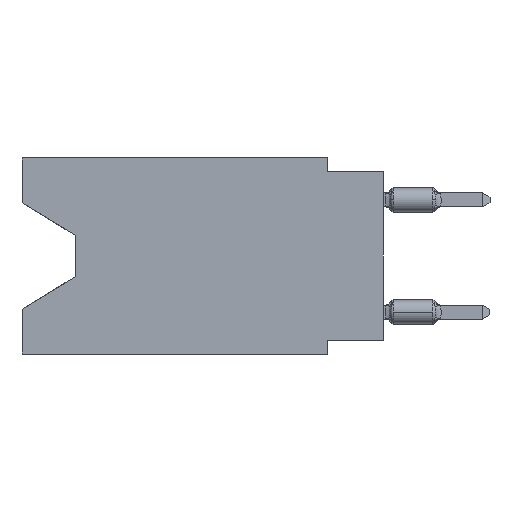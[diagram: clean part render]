
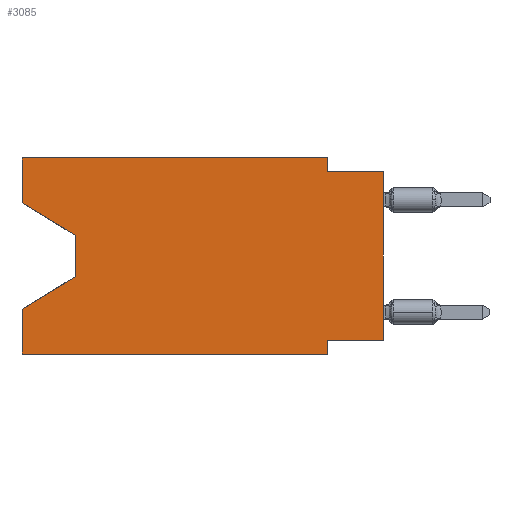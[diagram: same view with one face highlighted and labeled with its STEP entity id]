
A CAD part, left-side view. The second image highlights one B-rep face of the part: STEP entity #3085.
In plain terms, the highlighted planar face has unit normal (-1, 0, 0).
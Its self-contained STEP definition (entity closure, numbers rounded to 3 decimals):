
#282 = ORIENTED_EDGE ( 'NONE', *, *, #13436, .F. ) ;
#720 = LINE ( 'NONE', #1705, #8904 ) ;
#852 = EDGE_CURVE ( 'NONE', #2510, #11657, #2677, .T. ) ;
#994 = CARTESIAN_POINT ( 'NONE',  ( 0., 0., -8.255 ) ) ;
#1095 = LINE ( 'NONE', #13838, #10839 ) ;
#1414 = CARTESIAN_POINT ( 'NONE',  ( 0., 0., -0.635 ) ) ;
#1499 = ORIENTED_EDGE ( 'NONE', *, *, #11887, .F. ) ;
#1631 = ORIENTED_EDGE ( 'NONE', *, *, #2037, .T. ) ;
#1705 = CARTESIAN_POINT ( 'NONE',  ( 0., 16.383, -2.038 ) ) ;
#1725 = DIRECTION ( 'NONE',  ( 0., -1., 0. ) ) ;
#1851 = EDGE_CURVE ( 'NONE', #5161, #9197, #10149, .T. ) ;
#1967 = VERTEX_POINT ( 'NONE', #6021 ) ;
#1979 = DIRECTION ( 'NONE',  ( 0., 0., 1. ) ) ;
#2037 = EDGE_CURVE ( 'NONE', #12470, #5170, #7207, .T. ) ;
#2346 = DIRECTION ( 'NONE',  ( 0., 1., 0. ) ) ;
#2455 = ORIENTED_EDGE ( 'NONE', *, *, #5030, .T. ) ;
#2510 = VERTEX_POINT ( 'NONE', #6070 ) ;
#2540 = DIRECTION ( 'NONE',  ( 0., -1., 0. ) ) ;
#2578 = LINE ( 'NONE', #3625, #4548 ) ;
#2656 = DIRECTION ( 'NONE',  ( 0., 0., 1. ) ) ;
#2677 = LINE ( 'NONE', #13384, #4846 ) ;
#2776 = LINE ( 'NONE', #11307, #4141 ) ;
#2982 = EDGE_CURVE ( 'NONE', #5170, #8091, #7319, .T. ) ;
#3081 = CARTESIAN_POINT ( 'NONE',  ( 0., 16.383, -8.89 ) ) ;
#3085 = ADVANCED_FACE ( 'NONE', ( #8920 ), #7593, .F. ) ;
#3102 = EDGE_CURVE ( 'NONE', #3822, #9197, #7659, .T. ) ;
#3211 = AXIS2_PLACEMENT_3D ( 'NONE', #3523, #10937, #4641 ) ;
#3237 = DIRECTION ( 'NONE',  ( 0., 0., -1. ) ) ;
#3421 = ORIENTED_EDGE ( 'NONE', *, *, #4688, .T. ) ;
#3451 = VECTOR ( 'NONE', #2346, 1000. ) ;
#3523 = CARTESIAN_POINT ( 'NONE',  ( 0., 16.383, 0. ) ) ;
#3625 = CARTESIAN_POINT ( 'NONE',  ( 0., 2.54, -8.89 ) ) ;
#3763 = CARTESIAN_POINT ( 'NONE',  ( 0., 2.54, 0. ) ) ;
#3798 = DIRECTION ( 'NONE',  ( 0., -1., 0. ) ) ;
#3822 = VERTEX_POINT ( 'NONE', #11272 ) ;
#3915 = CARTESIAN_POINT ( 'NONE',  ( 0., 13.97, -3.505 ) ) ;
#4141 = VECTOR ( 'NONE', #1725, 1000. ) ;
#4416 = VERTEX_POINT ( 'NONE', #12717 ) ;
#4548 = VECTOR ( 'NONE', #10003, 1000. ) ;
#4641 = DIRECTION ( 'NONE',  ( 0., 0., -1. ) ) ;
#4688 = EDGE_CURVE ( 'NONE', #6809, #1967, #2776, .T. ) ;
#4715 = VERTEX_POINT ( 'NONE', #6003 ) ;
#4846 = VECTOR ( 'NONE', #3798, 1000. ) ;
#4956 = CARTESIAN_POINT ( 'NONE',  ( 0., 13.97, -3.505 ) ) ;
#5006 = VECTOR ( 'NONE', #2540, 1000. ) ;
#5030 = EDGE_CURVE ( 'NONE', #4715, #12470, #720, .T. ) ;
#5161 = VERTEX_POINT ( 'NONE', #994 ) ;
#5170 = VERTEX_POINT ( 'NONE', #5408 ) ;
#5408 = CARTESIAN_POINT ( 'NONE',  ( 0., 13.97, -5.385 ) ) ;
#5431 = CARTESIAN_POINT ( 'NONE',  ( 0., 0., -8.255 ) ) ;
#6003 = CARTESIAN_POINT ( 'NONE',  ( 0., 16.383, -2.038 ) ) ;
#6021 = CARTESIAN_POINT ( 'NONE',  ( 0., 2.54, -8.89 ) ) ;
#6070 = CARTESIAN_POINT ( 'NONE',  ( 0., 16.383, 0. ) ) ;
#6258 = CARTESIAN_POINT ( 'NONE',  ( 0., 13.97, -5.385 ) ) ;
#6510 = EDGE_CURVE ( 'NONE', #4715, #2510, #9610, .T. ) ;
#6740 = ORIENTED_EDGE ( 'NONE', *, *, #3102, .F. ) ;
#6809 = VERTEX_POINT ( 'NONE', #3081 ) ;
#7001 = CARTESIAN_POINT ( 'NONE',  ( 0., 0., 0. ) ) ;
#7096 = EDGE_CURVE ( 'NONE', #6809, #8091, #1095, .T. ) ;
#7201 = VECTOR ( 'NONE', #3237, 1000. ) ;
#7207 = LINE ( 'NONE', #4956, #12679 ) ;
#7319 = LINE ( 'NONE', #6258, #7476 ) ;
#7476 = VECTOR ( 'NONE', #13807, 1000. ) ;
#7593 = PLANE ( 'NONE',  #3211 ) ;
#7659 = LINE ( 'NONE', #1414, #5006 ) ;
#7849 = EDGE_LOOP ( 'NONE', ( #2455, #1631, #9806, #8907, #3421, #10992, #1499, #8838, #6740, #282, #10157, #9164 ) ) ;
#8091 = VERTEX_POINT ( 'NONE', #9621 ) ;
#8342 = VECTOR ( 'NONE', #2656, 1000. ) ;
#8394 = DIRECTION ( 'NONE',  ( 0., 0., 1. ) ) ;
#8727 = LINE ( 'NONE', #5431, #3451 ) ;
#8838 = ORIENTED_EDGE ( 'NONE', *, *, #1851, .T. ) ;
#8904 = VECTOR ( 'NONE', #10383, 1000. ) ;
#8907 = ORIENTED_EDGE ( 'NONE', *, *, #7096, .F. ) ;
#8920 = FACE_OUTER_BOUND ( 'NONE', #7849, .T. ) ;
#9164 = ORIENTED_EDGE ( 'NONE', *, *, #6510, .F. ) ;
#9197 = VERTEX_POINT ( 'NONE', #12702 ) ;
#9610 = LINE ( 'NONE', #11566, #10171 ) ;
#9621 = CARTESIAN_POINT ( 'NONE',  ( 0., 16.383, -6.852 ) ) ;
#9806 = ORIENTED_EDGE ( 'NONE', *, *, #2982, .T. ) ;
#10003 = DIRECTION ( 'NONE',  ( 0., 0., -1. ) ) ;
#10149 = LINE ( 'NONE', #7001, #8342 ) ;
#10157 = ORIENTED_EDGE ( 'NONE', *, *, #852, .F. ) ;
#10171 = VECTOR ( 'NONE', #1979, 1000. ) ;
#10383 = DIRECTION ( 'NONE',  ( 0., -0.855, -0.519 ) ) ;
#10839 = VECTOR ( 'NONE', #8394, 1000. ) ;
#10937 = DIRECTION ( 'NONE',  ( 1., 0., 0. ) ) ;
#10992 = ORIENTED_EDGE ( 'NONE', *, *, #11522, .F. ) ;
#11272 = CARTESIAN_POINT ( 'NONE',  ( 0., 2.54, -0.635 ) ) ;
#11307 = CARTESIAN_POINT ( 'NONE',  ( 0., 16.383, -8.89 ) ) ;
#11522 = EDGE_CURVE ( 'NONE', #4416, #1967, #2578, .T. ) ;
#11566 = CARTESIAN_POINT ( 'NONE',  ( 0., 16.383, 0. ) ) ;
#11657 = VERTEX_POINT ( 'NONE', #3763 ) ;
#11887 = EDGE_CURVE ( 'NONE', #5161, #4416, #8727, .T. ) ;
#12470 = VERTEX_POINT ( 'NONE', #3915 ) ;
#12679 = VECTOR ( 'NONE', #13709, 1000. ) ;
#12694 = CARTESIAN_POINT ( 'NONE',  ( 0., 2.54, 0. ) ) ;
#12702 = CARTESIAN_POINT ( 'NONE',  ( 0., 0., -0.635 ) ) ;
#12717 = CARTESIAN_POINT ( 'NONE',  ( 0., 2.54, -8.255 ) ) ;
#13384 = CARTESIAN_POINT ( 'NONE',  ( 0., 16.383, 0. ) ) ;
#13436 = EDGE_CURVE ( 'NONE', #11657, #3822, #13540, .T. ) ;
#13540 = LINE ( 'NONE', #12694, #7201 ) ;
#13709 = DIRECTION ( 'NONE',  ( 0., 0., -1. ) ) ;
#13807 = DIRECTION ( 'NONE',  ( 0., 0.855, -0.519 ) ) ;
#13838 = CARTESIAN_POINT ( 'NONE',  ( 0., 16.383, 0. ) ) ;
